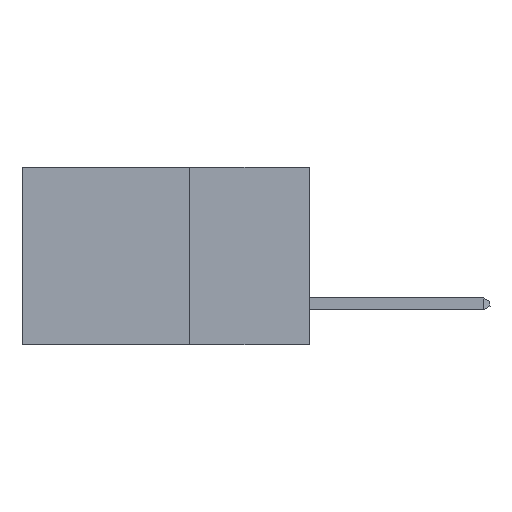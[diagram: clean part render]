
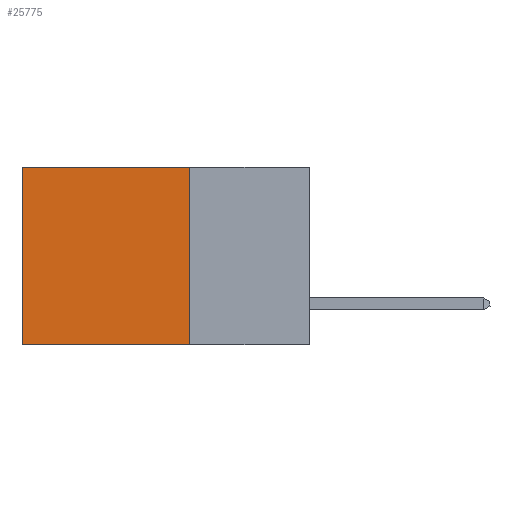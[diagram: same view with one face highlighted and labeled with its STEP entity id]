
A CAD part, left-side view. The second image highlights one B-rep face of the part: STEP entity #25775.
In plain terms, the highlighted planar face has unit normal (-1, 0, 0).
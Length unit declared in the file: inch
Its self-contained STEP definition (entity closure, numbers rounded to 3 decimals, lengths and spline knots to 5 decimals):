
#65 = ORIENTED_EDGE ( 'NONE', *, *, #33565, .T. ) ;
#564 = CARTESIAN_POINT ( 'NONE',  ( 0.2875, 0.25, 0. ) ) ;
#1036 = ORIENTED_EDGE ( 'NONE', *, *, #13569, .F. ) ;
#1275 = CARTESIAN_POINT ( 'NONE',  ( 0.2875, 0.25, 0. ) ) ;
#1451 = CARTESIAN_POINT ( 'NONE',  ( 0.2875, 0.25, -0.37 ) ) ;
#2748 = VECTOR ( 'NONE', #26746, 39.37008 ) ;
#4061 = DIRECTION ( 'NONE',  ( 0., 0., -1. ) ) ;
#4167 = DIRECTION ( 'NONE',  ( 1., 0., 0. ) ) ;
#4495 = VECTOR ( 'NONE', #4061, 39.37008 ) ;
#5204 = VERTEX_POINT ( 'NONE', #10630 ) ;
#7396 = EDGE_CURVE ( 'NONE', #5204, #35262, #28208, .T. ) ;
#10080 = EDGE_CURVE ( 'NONE', #27327, #10150, #30477, .T. ) ;
#10150 = VERTEX_POINT ( 'NONE', #15311 ) ;
#10630 = CARTESIAN_POINT ( 'NONE',  ( 0.2875, 0.6, 0. ) ) ;
#10892 = FACE_OUTER_BOUND ( 'NONE', #11900, .T. ) ;
#11900 = EDGE_LOOP ( 'NONE', ( #18565, #1036, #16717, #65 ) ) ;
#13569 = EDGE_CURVE ( 'NONE', #10150, #35262, #20742, .T. ) ;
#15311 = CARTESIAN_POINT ( 'NONE',  ( 0.2875, 0.25, -0.37 ) ) ;
#15764 = VECTOR ( 'NONE', #31544, 39.37008 ) ;
#16717 = ORIENTED_EDGE ( 'NONE', *, *, #10080, .F. ) ;
#17868 = PLANE ( 'NONE',  #19370 ) ;
#18565 = ORIENTED_EDGE ( 'NONE', *, *, #7396, .T. ) ;
#19370 = AXIS2_PLACEMENT_3D ( 'NONE', #1275, #4167, #23503 ) ;
#20539 = CARTESIAN_POINT ( 'NONE',  ( 0.2875, 0.25, 0. ) ) ;
#20742 = LINE ( 'NONE', #1451, #28086 ) ;
#23503 = DIRECTION ( 'NONE',  ( 0., 0., -1. ) ) ;
#23966 = LINE ( 'NONE', #35041, #2748 ) ;
#25775 = ADVANCED_FACE ( 'NONE', ( #10892 ), #17868, .F. ) ;
#26746 = DIRECTION ( 'NONE',  ( 0., 1., 0. ) ) ;
#27327 = VERTEX_POINT ( 'NONE', #564 ) ;
#28086 = VECTOR ( 'NONE', #34488, 39.37008 ) ;
#28208 = LINE ( 'NONE', #31583, #4495 ) ;
#29977 = CARTESIAN_POINT ( 'NONE',  ( 0.2875, 0.6, -0.37 ) ) ;
#30477 = LINE ( 'NONE', #20539, #15764 ) ;
#31544 = DIRECTION ( 'NONE',  ( 0., 0., -1. ) ) ;
#31583 = CARTESIAN_POINT ( 'NONE',  ( 0.2875, 0.6, 0. ) ) ;
#33565 = EDGE_CURVE ( 'NONE', #27327, #5204, #23966, .T. ) ;
#34488 = DIRECTION ( 'NONE',  ( 0., 1., 0. ) ) ;
#35041 = CARTESIAN_POINT ( 'NONE',  ( 0.2875, 0.25, 0. ) ) ;
#35262 = VERTEX_POINT ( 'NONE', #29977 ) ;
